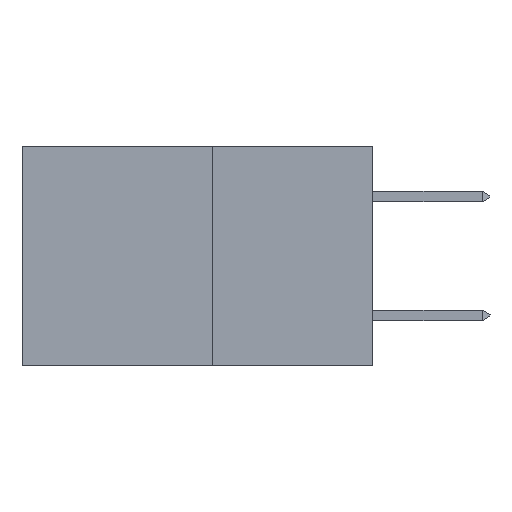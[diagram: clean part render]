
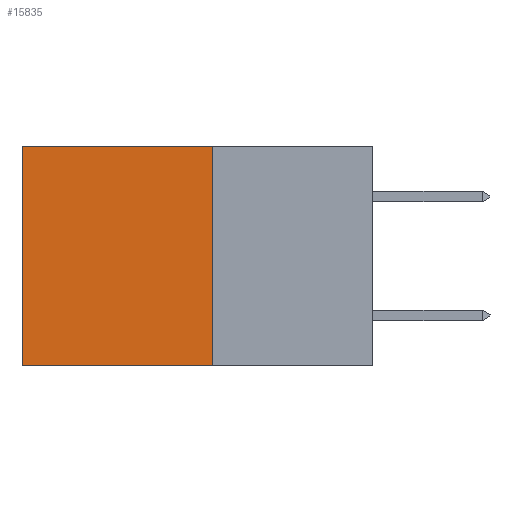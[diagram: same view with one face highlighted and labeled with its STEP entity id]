
A CAD part, left-side view. The second image highlights one B-rep face of the part: STEP entity #15835.
In plain terms, the highlighted planar face has unit normal (-1, 0, 0).
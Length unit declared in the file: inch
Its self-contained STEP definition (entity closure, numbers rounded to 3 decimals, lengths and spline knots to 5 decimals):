
#632 = VERTEX_POINT ( 'NONE', #13481 ) ;
#756 = CARTESIAN_POINT ( 'NONE',  ( 0.277, 0.59, -0.37 ) ) ;
#1401 = EDGE_CURVE ( 'NONE', #14726, #12010, #7812, .T. ) ;
#3699 = VECTOR ( 'NONE', #15707, 39.37008 ) ;
#4293 = EDGE_CURVE ( 'NONE', #14726, #632, #11500, .T. ) ;
#6122 = EDGE_CURVE ( 'NONE', #12010, #19657, #9132, .T. ) ;
#6435 = DIRECTION ( 'NONE',  ( 0., 0., -1. ) ) ;
#7136 = EDGE_LOOP ( 'NONE', ( #12394, #9621, #21218, #9193 ) ) ;
#7812 = LINE ( 'NONE', #9053, #16136 ) ;
#9053 = CARTESIAN_POINT ( 'NONE',  ( 0.277, 0.27, -0.37 ) ) ;
#9125 = VECTOR ( 'NONE', #21415, 39.37008 ) ;
#9132 = LINE ( 'NONE', #18240, #3699 ) ;
#9193 = ORIENTED_EDGE ( 'NONE', *, *, #4293, .T. ) ;
#9621 = ORIENTED_EDGE ( 'NONE', *, *, #6122, .F. ) ;
#10034 = DIRECTION ( 'NONE',  ( 0., 1., 0. ) ) ;
#10630 = DIRECTION ( 'NONE',  ( 0., 0., -1. ) ) ;
#10739 = CARTESIAN_POINT ( 'NONE',  ( 0.277, 0.27, 0. ) ) ;
#11500 = LINE ( 'NONE', #10739, #20234 ) ;
#12010 = VERTEX_POINT ( 'NONE', #15636 ) ;
#12394 = ORIENTED_EDGE ( 'NONE', *, *, #19315, .T. ) ;
#13481 = CARTESIAN_POINT ( 'NONE',  ( 0.277, 0.59, 0. ) ) ;
#14108 = CARTESIAN_POINT ( 'NONE',  ( 0.277, 0.27, -0.37 ) ) ;
#14726 = VERTEX_POINT ( 'NONE', #20144 ) ;
#15636 = CARTESIAN_POINT ( 'NONE',  ( 0.277, 0.27, -0.37 ) ) ;
#15707 = DIRECTION ( 'NONE',  ( 0., 1., 0. ) ) ;
#15835 = ADVANCED_FACE ( 'NONE', ( #18876 ), #17626, .F. ) ;
#16136 = VECTOR ( 'NONE', #6435, 39.37008 ) ;
#17626 = PLANE ( 'NONE',  #20315 ) ;
#18240 = CARTESIAN_POINT ( 'NONE',  ( 0.277, 0.27, -0.37 ) ) ;
#18876 = FACE_OUTER_BOUND ( 'NONE', #7136, .T. ) ;
#19315 = EDGE_CURVE ( 'NONE', #632, #19657, #22522, .T. ) ;
#19657 = VERTEX_POINT ( 'NONE', #756 ) ;
#19687 = CARTESIAN_POINT ( 'NONE',  ( 0.277, 0.59, -0.37 ) ) ;
#20144 = CARTESIAN_POINT ( 'NONE',  ( 0.277, 0.27, 0. ) ) ;
#20234 = VECTOR ( 'NONE', #10034, 39.37008 ) ;
#20315 = AXIS2_PLACEMENT_3D ( 'NONE', #14108, #21085, #10630 ) ;
#21085 = DIRECTION ( 'NONE',  ( 1., 0., 0. ) ) ;
#21218 = ORIENTED_EDGE ( 'NONE', *, *, #1401, .F. ) ;
#21415 = DIRECTION ( 'NONE',  ( 0., 0., -1. ) ) ;
#22522 = LINE ( 'NONE', #19687, #9125 ) ;
